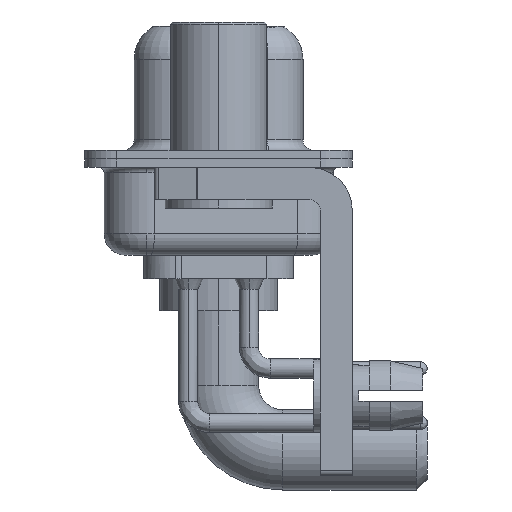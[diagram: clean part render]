
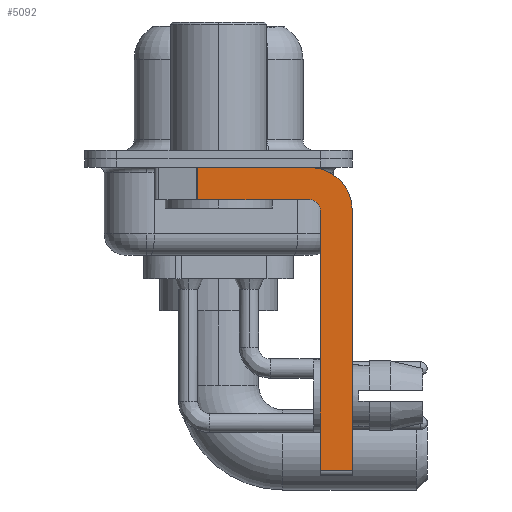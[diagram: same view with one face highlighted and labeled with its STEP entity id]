
A CAD part, left-side view. The second image highlights one B-rep face of the part: STEP entity #5092.
In plain terms, the highlighted planar face has unit normal (-1, 0, 0).
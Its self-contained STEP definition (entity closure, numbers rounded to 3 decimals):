
#202 = CARTESIAN_POINT ( 'NONE',  ( -2.9, -6.25, -14.55 ) ) ;
#236 = CARTESIAN_POINT ( 'NONE',  ( -2.9, -6.25, -2.4 ) ) ;
#1216 = VECTOR ( 'NONE', #14452, 1000. ) ;
#2122 = VECTOR ( 'NONE', #26048, 1000. ) ;
#3327 = CARTESIAN_POINT ( 'NONE',  ( -2.9, 0.978, -1.9 ) ) ;
#3641 = EDGE_CURVE ( 'NONE', #12052, #7572, #16147, .T. ) ;
#3974 = LINE ( 'NONE', #5845, #17729 ) ;
#4705 = AXIS2_PLACEMENT_3D ( 'NONE', #24725, #14546, #6866 ) ;
#4828 = CARTESIAN_POINT ( 'NONE',  ( -2.9, -4.75, -2.4 ) ) ;
#4964 = VERTEX_POINT ( 'NONE', #11685 ) ;
#5057 = LINE ( 'NONE', #3327, #11012 ) ;
#5092 = ADVANCED_FACE ( 'NONE', ( #13942 ), #12082, .F. ) ;
#5201 = VERTEX_POINT ( 'NONE', #236 ) ;
#5641 = VERTEX_POINT ( 'NONE', #202 ) ;
#5845 = CARTESIAN_POINT ( 'NONE',  ( -2.9, -4.75, -14.8 ) ) ;
#5963 = CARTESIAN_POINT ( 'NONE',  ( -2.9, -4.25, -1.9 ) ) ;
#6193 = CARTESIAN_POINT ( 'NONE',  ( -2.9, 3., -0.4 ) ) ;
#6581 = DIRECTION ( 'NONE',  ( 0., -1., 0. ) ) ;
#6655 = EDGE_CURVE ( 'NONE', #22760, #12052, #3974, .T. ) ;
#6866 = DIRECTION ( 'NONE',  ( 0., 0., 1. ) ) ;
#6887 = LINE ( 'NONE', #12866, #1216 ) ;
#7045 = DIRECTION ( 'NONE',  ( 0., 1., 0. ) ) ;
#7428 = VECTOR ( 'NONE', #6581, 1000. ) ;
#7572 = VERTEX_POINT ( 'NONE', #5963 ) ;
#7999 = ORIENTED_EDGE ( 'NONE', *, *, #17587, .T. ) ;
#8362 = VECTOR ( 'NONE', #7045, 1000. ) ;
#8444 = CIRCLE ( 'NONE', #24456, 2. ) ;
#8828 = EDGE_CURVE ( 'NONE', #18327, #4964, #5057, .T. ) ;
#8996 = ORIENTED_EDGE ( 'NONE', *, *, #6655, .F. ) ;
#9406 = EDGE_CURVE ( 'NONE', #5201, #5641, #11534, .T. ) ;
#9493 = CARTESIAN_POINT ( 'NONE',  ( -2.9, -4.25, -2.4 ) ) ;
#9516 = ORIENTED_EDGE ( 'NONE', *, *, #3641, .F. ) ;
#11012 = VECTOR ( 'NONE', #21482, 1000. ) ;
#11045 = EDGE_CURVE ( 'NONE', #18327, #12298, #18794, .T. ) ;
#11175 = LINE ( 'NONE', #13422, #8362 ) ;
#11534 = LINE ( 'NONE', #23842, #2122 ) ;
#11685 = CARTESIAN_POINT ( 'NONE',  ( -2.9, 0.978, -1.9 ) ) ;
#12052 = VERTEX_POINT ( 'NONE', #4828 ) ;
#12082 = PLANE ( 'NONE',  #14682 ) ;
#12124 = EDGE_LOOP ( 'NONE', ( #18060, #26053, #18147, #9516, #8996, #7999, #13377, #26000 ) ) ;
#12298 = VERTEX_POINT ( 'NONE', #18831 ) ;
#12866 = CARTESIAN_POINT ( 'NONE',  ( -2.9, -4.25, -14.55 ) ) ;
#13377 = ORIENTED_EDGE ( 'NONE', *, *, #9406, .F. ) ;
#13422 = CARTESIAN_POINT ( 'NONE',  ( -2.9, -4.25, -1.9 ) ) ;
#13942 = FACE_OUTER_BOUND ( 'NONE', #12124, .T. ) ;
#14182 = DIRECTION ( 'NONE',  ( 1., 0., 0. ) ) ;
#14452 = DIRECTION ( 'NONE',  ( 0., -1., 0. ) ) ;
#14546 = DIRECTION ( 'NONE',  ( -1., 0., 0. ) ) ;
#14580 = EDGE_CURVE ( 'NONE', #7572, #4964, #11175, .T. ) ;
#14682 = AXIS2_PLACEMENT_3D ( 'NONE', #17794, #14182, #20150 ) ;
#14898 = CARTESIAN_POINT ( 'NONE',  ( -2.9, 0.978, -0.4 ) ) ;
#16147 = CIRCLE ( 'NONE', #4705, 0.5 ) ;
#17174 = DIRECTION ( 'NONE',  ( 1., 0., 0. ) ) ;
#17570 = DIRECTION ( 'NONE',  ( 0., 0., -1. ) ) ;
#17587 = EDGE_CURVE ( 'NONE', #22760, #5641, #6887, .T. ) ;
#17729 = VECTOR ( 'NONE', #18182, 1000. ) ;
#17794 = CARTESIAN_POINT ( 'NONE',  ( -2.9, -4.25, -2.4 ) ) ;
#18060 = ORIENTED_EDGE ( 'NONE', *, *, #11045, .F. ) ;
#18147 = ORIENTED_EDGE ( 'NONE', *, *, #14580, .F. ) ;
#18182 = DIRECTION ( 'NONE',  ( 0., 0., 1. ) ) ;
#18327 = VERTEX_POINT ( 'NONE', #14898 ) ;
#18794 = LINE ( 'NONE', #6193, #7428 ) ;
#18831 = CARTESIAN_POINT ( 'NONE',  ( -2.9, -4.25, -0.4 ) ) ;
#20150 = DIRECTION ( 'NONE',  ( 0., 0., -1. ) ) ;
#21482 = DIRECTION ( 'NONE',  ( 0., 0., -1. ) ) ;
#22507 = EDGE_CURVE ( 'NONE', #12298, #5201, #8444, .T. ) ;
#22760 = VERTEX_POINT ( 'NONE', #23797 ) ;
#23797 = CARTESIAN_POINT ( 'NONE',  ( -2.9, -4.75, -14.55 ) ) ;
#23842 = CARTESIAN_POINT ( 'NONE',  ( -2.9, -6.25, -2.4 ) ) ;
#24456 = AXIS2_PLACEMENT_3D ( 'NONE', #9493, #17174, #17570 ) ;
#24725 = CARTESIAN_POINT ( 'NONE',  ( -2.9, -4.25, -2.4 ) ) ;
#26000 = ORIENTED_EDGE ( 'NONE', *, *, #22507, .F. ) ;
#26048 = DIRECTION ( 'NONE',  ( 0., 0., -1. ) ) ;
#26053 = ORIENTED_EDGE ( 'NONE', *, *, #8828, .T. ) ;
